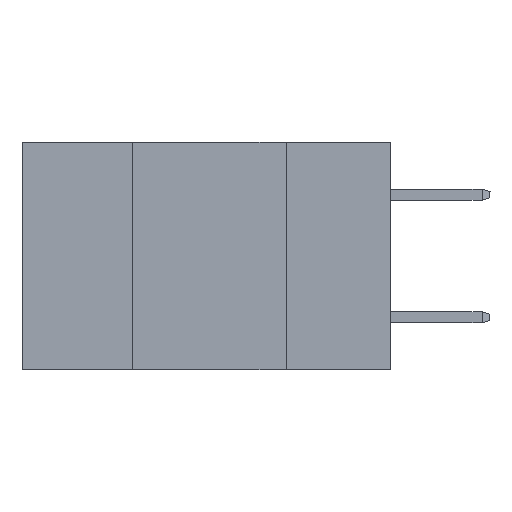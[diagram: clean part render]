
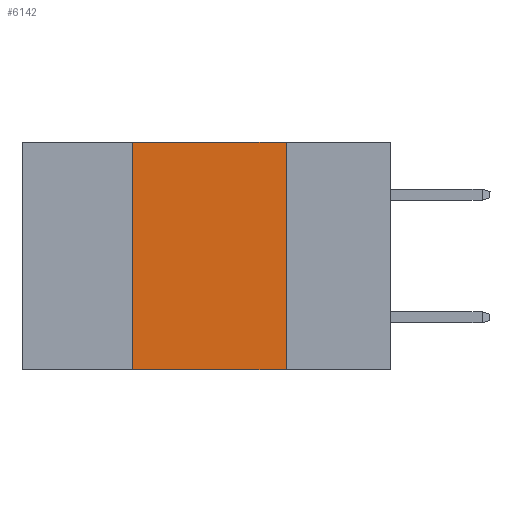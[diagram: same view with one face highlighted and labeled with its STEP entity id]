
A CAD part, left-side view. The second image highlights one B-rep face of the part: STEP entity #6142.
In plain terms, the highlighted planar face has unit normal (-1, 0, 0).
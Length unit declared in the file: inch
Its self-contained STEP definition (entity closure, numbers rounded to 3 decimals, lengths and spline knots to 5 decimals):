
#113 = CARTESIAN_POINT ( 'NONE',  ( 0., 0.17, 0. ) ) ;
#369 = ORIENTED_EDGE ( 'NONE', *, *, #13967, .T. ) ;
#439 = DIRECTION ( 'NONE',  ( 1., 0., 0. ) ) ;
#544 = CARTESIAN_POINT ( 'NONE',  ( 0., 0.6, 0. ) ) ;
#562 = LINE ( 'NONE', #6596, #17893 ) ;
#621 = ORIENTED_EDGE ( 'NONE', *, *, #15676, .F. ) ;
#1568 = DIRECTION ( 'NONE',  ( 0., -1., 0. ) ) ;
#2396 = VECTOR ( 'NONE', #1568, 39.37008 ) ;
#3717 = VERTEX_POINT ( 'NONE', #16037 ) ;
#5028 = DIRECTION ( 'NONE',  ( 0., 0., 1. ) ) ;
#6142 = ADVANCED_FACE ( 'NONE', ( #9418 ), #10541, .F. ) ;
#6596 = CARTESIAN_POINT ( 'NONE',  ( 0., 0.42, 0. ) ) ;
#6845 = CARTESIAN_POINT ( 'NONE',  ( 0., 0.17, 0. ) ) ;
#6867 = EDGE_LOOP ( 'NONE', ( #14658, #621, #9849, #369 ) ) ;
#7337 = VECTOR ( 'NONE', #10354, 39.37008 ) ;
#8586 = VERTEX_POINT ( 'NONE', #6845 ) ;
#8854 = DIRECTION ( 'NONE',  ( 0., 0., -1. ) ) ;
#9418 = FACE_OUTER_BOUND ( 'NONE', #6867, .T. ) ;
#9849 = ORIENTED_EDGE ( 'NONE', *, *, #18092, .F. ) ;
#10185 = VERTEX_POINT ( 'NONE', #10877 ) ;
#10354 = DIRECTION ( 'NONE',  ( 0., -1., 0. ) ) ;
#10541 = PLANE ( 'NONE',  #15285 ) ;
#10573 = CARTESIAN_POINT ( 'NONE',  ( 0., 0.6, 0. ) ) ;
#10877 = CARTESIAN_POINT ( 'NONE',  ( 0., 0.17, -0.37 ) ) ;
#11830 = CARTESIAN_POINT ( 'NONE',  ( 0., 0.6, -0.37 ) ) ;
#12028 = LINE ( 'NONE', #11830, #7337 ) ;
#12132 = VERTEX_POINT ( 'NONE', #13496 ) ;
#12234 = LINE ( 'NONE', #10573, #2396 ) ;
#13403 = DIRECTION ( 'NONE',  ( 0., 0., -1. ) ) ;
#13496 = CARTESIAN_POINT ( 'NONE',  ( 0., 0.42, -0.37 ) ) ;
#13967 = EDGE_CURVE ( 'NONE', #12132, #10185, #12028, .T. ) ;
#14658 = ORIENTED_EDGE ( 'NONE', *, *, #15773, .F. ) ;
#15285 = AXIS2_PLACEMENT_3D ( 'NONE', #544, #439, #8854 ) ;
#15676 = EDGE_CURVE ( 'NONE', #3717, #8586, #12234, .T. ) ;
#15773 = EDGE_CURVE ( 'NONE', #8586, #10185, #17798, .T. ) ;
#16037 = CARTESIAN_POINT ( 'NONE',  ( 0., 0.42, 0. ) ) ;
#17697 = VECTOR ( 'NONE', #13403, 39.37008 ) ;
#17798 = LINE ( 'NONE', #113, #17697 ) ;
#17893 = VECTOR ( 'NONE', #5028, 39.37008 ) ;
#18092 = EDGE_CURVE ( 'NONE', #12132, #3717, #562, .T. ) ;
